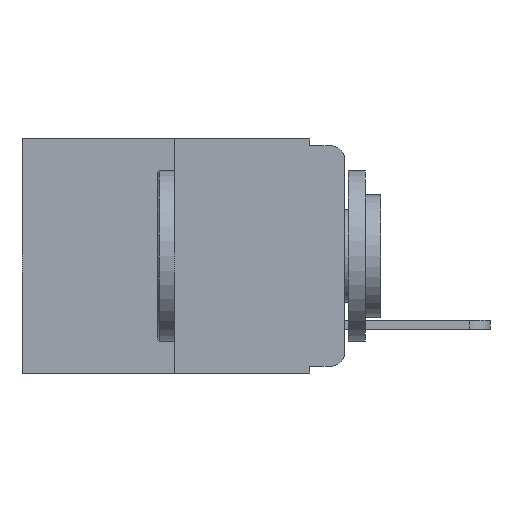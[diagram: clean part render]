
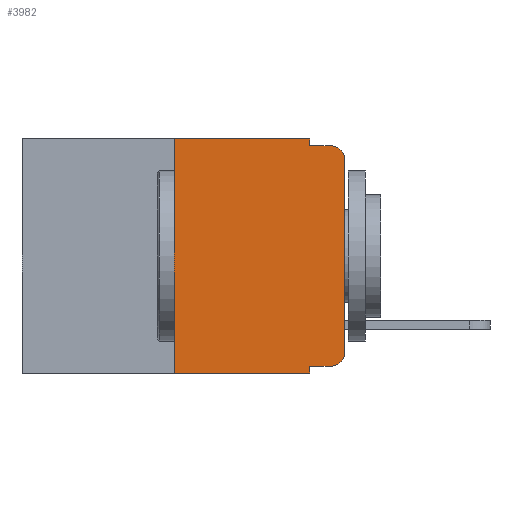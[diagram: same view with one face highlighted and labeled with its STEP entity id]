
A CAD part, left-side view. The second image highlights one B-rep face of the part: STEP entity #3982.
In plain terms, the highlighted planar face has unit normal (-1, 0, 0).
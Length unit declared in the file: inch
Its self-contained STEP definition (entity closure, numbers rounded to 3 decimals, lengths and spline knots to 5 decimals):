
#143 = DIRECTION ( 'NONE',  ( 0., 0., -1. ) ) ;
#187 = LINE ( 'NONE', #9147, #11070 ) ;
#352 = VECTOR ( 'NONE', #3657, 39.37008 ) ;
#496 = LINE ( 'NONE', #11948, #352 ) ;
#611 = CARTESIAN_POINT ( 'NONE',  ( 0., 0.02, -0.03 ) ) ;
#729 = AXIS2_PLACEMENT_3D ( 'NONE', #6952, #2432, #7035 ) ;
#950 = VERTEX_POINT ( 'NONE', #8839 ) ;
#1055 = CARTESIAN_POINT ( 'NONE',  ( 0., 0.051, 0. ) ) ;
#1185 = CARTESIAN_POINT ( 'NONE',  ( 0., 0.25, 0. ) ) ;
#1189 = EDGE_CURVE ( 'NONE', #950, #5153, #9265, .T. ) ;
#1815 = FACE_OUTER_BOUND ( 'NONE', #4868, .T. ) ;
#1902 = AXIS2_PLACEMENT_3D ( 'NONE', #611, #6244, #6281 ) ;
#2056 = CARTESIAN_POINT ( 'NONE',  ( 0., 0.02, -0.333 ) ) ;
#2079 = CARTESIAN_POINT ( 'NONE',  ( 0., 0.02, -0.01 ) ) ;
#2113 = CARTESIAN_POINT ( 'NONE',  ( 0., 0., -0.03 ) ) ;
#2121 = DIRECTION ( 'NONE',  ( 0., 0., 1. ) ) ;
#2301 = EDGE_CURVE ( 'NONE', #8626, #10393, #2750, .T. ) ;
#2432 = DIRECTION ( 'NONE',  ( 1., 0., 0. ) ) ;
#2439 = ORIENTED_EDGE ( 'NONE', *, *, #2301, .T. ) ;
#2750 = CIRCLE ( 'NONE', #1902, 0.02 ) ;
#2843 = VECTOR ( 'NONE', #10760, 39.37008 ) ;
#2863 = VECTOR ( 'NONE', #143, 39.37008 ) ;
#3008 = CARTESIAN_POINT ( 'NONE',  ( 0., 0.02, -0.313 ) ) ;
#3083 = VERTEX_POINT ( 'NONE', #5587 ) ;
#3200 = VERTEX_POINT ( 'NONE', #5775 ) ;
#3226 = EDGE_CURVE ( 'NONE', #9326, #7735, #10216, .T. ) ;
#3359 = DIRECTION ( 'NONE',  ( 0., -1., 0. ) ) ;
#3657 = DIRECTION ( 'NONE',  ( 0., -1., 0. ) ) ;
#3982 = ADVANCED_FACE ( 'NONE', ( #1815 ), #8056, .F. ) ;
#4184 = EDGE_CURVE ( 'NONE', #3200, #10716, #187, .T. ) ;
#4266 = CARTESIAN_POINT ( 'NONE',  ( 0., 0.051, 0. ) ) ;
#4270 = VERTEX_POINT ( 'NONE', #2056 ) ;
#4391 = ORIENTED_EDGE ( 'NONE', *, *, #11028, .F. ) ;
#4454 = VECTOR ( 'NONE', #7320, 39.37008 ) ;
#4542 = ORIENTED_EDGE ( 'NONE', *, *, #1189, .F. ) ;
#4787 = EDGE_CURVE ( 'NONE', #3200, #4270, #7262, .T. ) ;
#4868 = EDGE_LOOP ( 'NONE', ( #6155, #2439, #9780, #7606, #4391, #4542, #11443, #11639, #11573, #8527 ) ) ;
#5027 = CARTESIAN_POINT ( 'NONE',  ( 0., 0.051, -0.01 ) ) ;
#5153 = VERTEX_POINT ( 'NONE', #1185 ) ;
#5196 = EDGE_CURVE ( 'NONE', #3083, #8626, #8133, .T. ) ;
#5301 = EDGE_CURVE ( 'NONE', #7735, #10393, #10043, .T. ) ;
#5587 = CARTESIAN_POINT ( 'NONE',  ( 0., 0., -0.313 ) ) ;
#5775 = CARTESIAN_POINT ( 'NONE',  ( 0., 0.051, -0.333 ) ) ;
#5997 = VECTOR ( 'NONE', #3359, 39.37008 ) ;
#6155 = ORIENTED_EDGE ( 'NONE', *, *, #5196, .T. ) ;
#6244 = DIRECTION ( 'NONE',  ( -1., 0., 0. ) ) ;
#6281 = DIRECTION ( 'NONE',  ( 0., 0., -1. ) ) ;
#6376 = CARTESIAN_POINT ( 'NONE',  ( 0., 0.25, 0. ) ) ;
#6535 = VECTOR ( 'NONE', #12112, 39.37008 ) ;
#6952 = CARTESIAN_POINT ( 'NONE',  ( 0., 0.473, 0. ) ) ;
#7035 = DIRECTION ( 'NONE',  ( 0., 0., -1. ) ) ;
#7144 = DIRECTION ( 'NONE',  ( 0., 0., -1. ) ) ;
#7262 = LINE ( 'NONE', #10311, #6535 ) ;
#7320 = DIRECTION ( 'NONE',  ( 0., 0., 1. ) ) ;
#7472 = AXIS2_PLACEMENT_3D ( 'NONE', #3008, #8678, #9667 ) ;
#7606 = ORIENTED_EDGE ( 'NONE', *, *, #3226, .F. ) ;
#7735 = VERTEX_POINT ( 'NONE', #5027 ) ;
#8056 = PLANE ( 'NONE',  #729 ) ;
#8133 = LINE ( 'NONE', #9591, #10495 ) ;
#8494 = LINE ( 'NONE', #8917, #5997 ) ;
#8527 = ORIENTED_EDGE ( 'NONE', *, *, #11654, .T. ) ;
#8626 = VERTEX_POINT ( 'NONE', #2113 ) ;
#8678 = DIRECTION ( 'NONE',  ( -1., 0., 0. ) ) ;
#8839 = CARTESIAN_POINT ( 'NONE',  ( 0., 0.25, -0.343 ) ) ;
#8917 = CARTESIAN_POINT ( 'NONE',  ( 0., 0.473, -0.343 ) ) ;
#8969 = EDGE_CURVE ( 'NONE', #950, #10716, #8494, .T. ) ;
#9147 = CARTESIAN_POINT ( 'NONE',  ( 0., 0.051, 0. ) ) ;
#9265 = LINE ( 'NONE', #6376, #4454 ) ;
#9326 = VERTEX_POINT ( 'NONE', #4266 ) ;
#9591 = CARTESIAN_POINT ( 'NONE',  ( 0., 0., 0. ) ) ;
#9667 = DIRECTION ( 'NONE',  ( 0., 0., -1. ) ) ;
#9780 = ORIENTED_EDGE ( 'NONE', *, *, #5301, .F. ) ;
#9892 = CARTESIAN_POINT ( 'NONE',  ( 0., 0.051, -0.343 ) ) ;
#10043 = LINE ( 'NONE', #10717, #2843 ) ;
#10082 = CIRCLE ( 'NONE', #7472, 0.02 ) ;
#10216 = LINE ( 'NONE', #1055, #2863 ) ;
#10311 = CARTESIAN_POINT ( 'NONE',  ( 0., 0.051, -0.333 ) ) ;
#10393 = VERTEX_POINT ( 'NONE', #2079 ) ;
#10495 = VECTOR ( 'NONE', #2121, 39.37008 ) ;
#10716 = VERTEX_POINT ( 'NONE', #9892 ) ;
#10717 = CARTESIAN_POINT ( 'NONE',  ( 0., 0.051, -0.01 ) ) ;
#10760 = DIRECTION ( 'NONE',  ( 0., -1., 0. ) ) ;
#11028 = EDGE_CURVE ( 'NONE', #5153, #9326, #496, .T. ) ;
#11070 = VECTOR ( 'NONE', #7144, 39.37008 ) ;
#11443 = ORIENTED_EDGE ( 'NONE', *, *, #8969, .T. ) ;
#11573 = ORIENTED_EDGE ( 'NONE', *, *, #4787, .T. ) ;
#11639 = ORIENTED_EDGE ( 'NONE', *, *, #4184, .F. ) ;
#11654 = EDGE_CURVE ( 'NONE', #4270, #3083, #10082, .T. ) ;
#11948 = CARTESIAN_POINT ( 'NONE',  ( 0., 0.473, 0. ) ) ;
#12112 = DIRECTION ( 'NONE',  ( 0., -1., 0. ) ) ;
